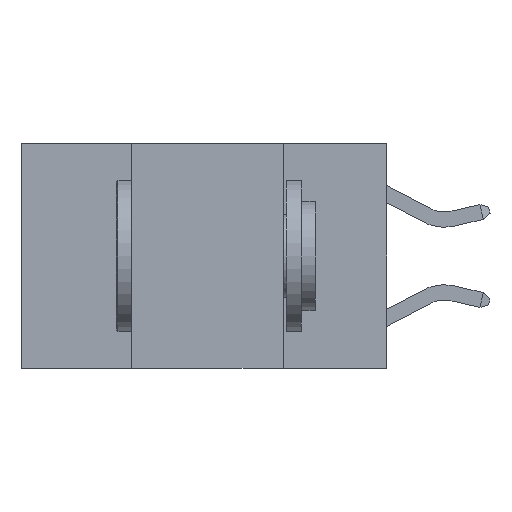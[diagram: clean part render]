
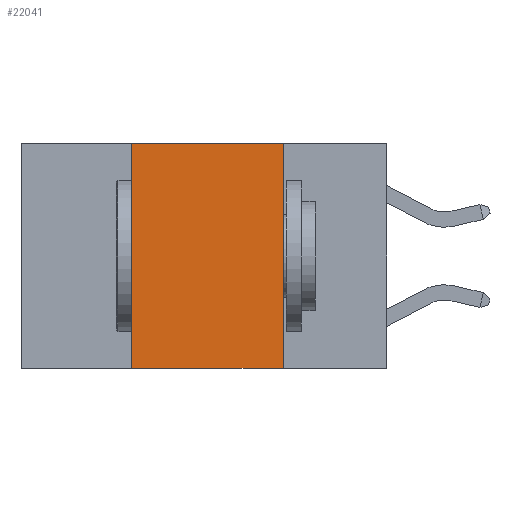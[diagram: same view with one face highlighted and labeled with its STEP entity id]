
A CAD part, left-side view. The second image highlights one B-rep face of the part: STEP entity #22041.
In plain terms, the highlighted planar face has unit normal (-1, 0, 0).
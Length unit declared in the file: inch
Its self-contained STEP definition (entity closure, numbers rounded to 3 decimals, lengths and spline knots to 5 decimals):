
#196 = VERTEX_POINT ( 'NONE', #18808 ) ;
#1649 = VECTOR ( 'NONE', #7215, 39.37008 ) ;
#1982 = PLANE ( 'NONE',  #8577 ) ;
#2291 = CARTESIAN_POINT ( 'NONE',  ( 0., 0.42, 0. ) ) ;
#4321 = LINE ( 'NONE', #11468, #1649 ) ;
#4903 = ORIENTED_EDGE ( 'NONE', *, *, #19038, .T. ) ;
#6405 = VERTEX_POINT ( 'NONE', #22060 ) ;
#7215 = DIRECTION ( 'NONE',  ( 0., -1., 0. ) ) ;
#7558 = LINE ( 'NONE', #17325, #31156 ) ;
#8163 = ORIENTED_EDGE ( 'NONE', *, *, #10786, .F. ) ;
#8577 = AXIS2_PLACEMENT_3D ( 'NONE', #14650, #31920, #27249 ) ;
#8843 = DIRECTION ( 'NONE',  ( 0., -1., 0. ) ) ;
#10503 = CARTESIAN_POINT ( 'NONE',  ( 0., 0.42, 0. ) ) ;
#10786 = EDGE_CURVE ( 'NONE', #31101, #6405, #11752, .T. ) ;
#11468 = CARTESIAN_POINT ( 'NONE',  ( 0., 0.6, -0.37 ) ) ;
#11752 = LINE ( 'NONE', #23781, #15958 ) ;
#14650 = CARTESIAN_POINT ( 'NONE',  ( 0., 0.6, 0. ) ) ;
#15958 = VECTOR ( 'NONE', #8843, 39.37008 ) ;
#16133 = VERTEX_POINT ( 'NONE', #21297 ) ;
#17325 = CARTESIAN_POINT ( 'NONE',  ( 0., 0.17, 0. ) ) ;
#18739 = EDGE_CURVE ( 'NONE', #16133, #31101, #30088, .T. ) ;
#18808 = CARTESIAN_POINT ( 'NONE',  ( 0., 0.17, -0.37 ) ) ;
#18879 = ORIENTED_EDGE ( 'NONE', *, *, #18739, .F. ) ;
#19038 = EDGE_CURVE ( 'NONE', #16133, #196, #4321, .T. ) ;
#20812 = VECTOR ( 'NONE', #29764, 39.37008 ) ;
#21297 = CARTESIAN_POINT ( 'NONE',  ( 0., 0.42, -0.37 ) ) ;
#22041 = ADVANCED_FACE ( 'NONE', ( #24369 ), #1982, .F. ) ;
#22060 = CARTESIAN_POINT ( 'NONE',  ( 0., 0.17, 0. ) ) ;
#23781 = CARTESIAN_POINT ( 'NONE',  ( 0., 0.6, 0. ) ) ;
#24369 = FACE_OUTER_BOUND ( 'NONE', #28457, .T. ) ;
#24583 = EDGE_CURVE ( 'NONE', #6405, #196, #7558, .T. ) ;
#27249 = DIRECTION ( 'NONE',  ( 0., 0., -1. ) ) ;
#28457 = EDGE_LOOP ( 'NONE', ( #31331, #8163, #18879, #4903 ) ) ;
#29764 = DIRECTION ( 'NONE',  ( 0., 0., 1. ) ) ;
#30088 = LINE ( 'NONE', #10503, #20812 ) ;
#30405 = DIRECTION ( 'NONE',  ( 0., 0., -1. ) ) ;
#31101 = VERTEX_POINT ( 'NONE', #2291 ) ;
#31156 = VECTOR ( 'NONE', #30405, 39.37008 ) ;
#31331 = ORIENTED_EDGE ( 'NONE', *, *, #24583, .F. ) ;
#31920 = DIRECTION ( 'NONE',  ( 1., 0., 0. ) ) ;
